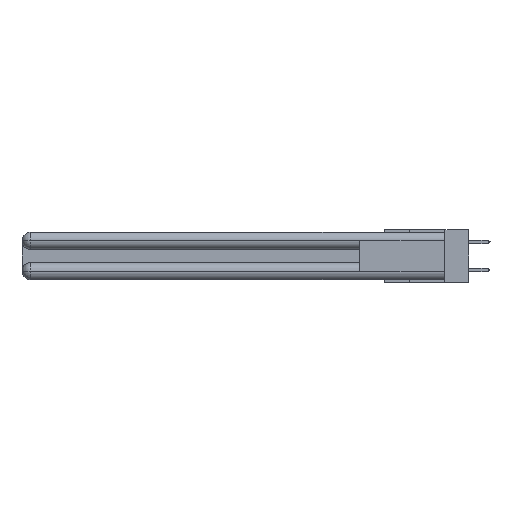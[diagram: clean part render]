
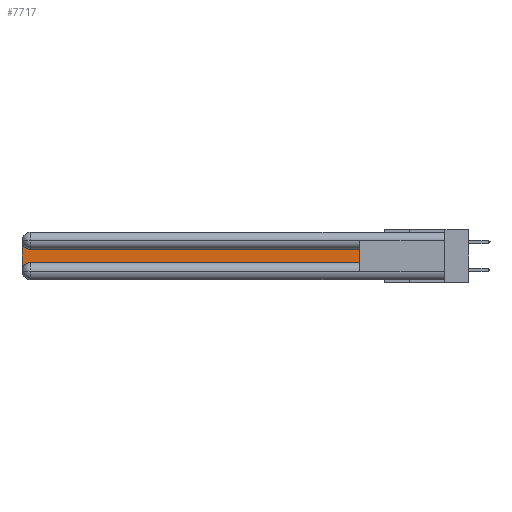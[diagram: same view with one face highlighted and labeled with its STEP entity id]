
A CAD part, left-side view. The second image highlights one B-rep face of the part: STEP entity #7717.
In plain terms, the highlighted planar face has unit normal (-1, 0, 0).
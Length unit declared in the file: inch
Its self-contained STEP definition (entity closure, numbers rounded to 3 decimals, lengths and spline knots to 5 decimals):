
#254 = DIRECTION ( 'NONE',  ( 0., 0., -1. ) ) ;
#842 = VECTOR ( 'NONE', #1793, 39.37008 ) ;
#943 = VERTEX_POINT ( 'NONE', #5503 ) ;
#1793 = DIRECTION ( 'NONE',  ( 0., 0., 1. ) ) ;
#3448 = CARTESIAN_POINT ( 'NONE',  ( 0.075, 0.6, -0.2175 ) ) ;
#3999 = DIRECTION ( 'NONE',  ( 0., 1., 0. ) ) ;
#5503 = CARTESIAN_POINT ( 'NONE',  ( 0.075, 0.6, -0.1225 ) ) ;
#5796 = DIRECTION ( 'NONE',  ( 0., 0., -1. ) ) ;
#7717 = ADVANCED_FACE ( 'NONE', ( #32579 ), #22457, .F. ) ;
#8227 = ORIENTED_EDGE ( 'NONE', *, *, #26157, .T. ) ;
#8641 = VECTOR ( 'NONE', #36005, 39.37008 ) ;
#8813 = AXIS2_PLACEMENT_3D ( 'NONE', #33532, #16880, #254 ) ;
#9236 = VERTEX_POINT ( 'NONE', #13924 ) ;
#10977 = VERTEX_POINT ( 'NONE', #3448 ) ;
#12655 = ORIENTED_EDGE ( 'NONE', *, *, #34220, .T. ) ;
#13216 = AXIS2_PLACEMENT_3D ( 'NONE', #22332, #30378, #13701 ) ;
#13701 = DIRECTION ( 'NONE',  ( 0., 0., -1. ) ) ;
#13829 = CARTESIAN_POINT ( 'NONE',  ( 0.075, 3., -0.1225 ) ) ;
#13924 = CARTESIAN_POINT ( 'NONE',  ( 0.075, 2.94, -0.1225 ) ) ;
#15434 = LINE ( 'NONE', #25744, #21072 ) ;
#16880 = DIRECTION ( 'NONE',  ( 1., 0., 0. ) ) ;
#17345 = CIRCLE ( 'NONE', #13216, 0.06 ) ;
#17694 = ORIENTED_EDGE ( 'NONE', *, *, #28349, .T. ) ;
#17769 = CARTESIAN_POINT ( 'NONE',  ( 0.075, 0.6, -0.1225 ) ) ;
#18044 = ORIENTED_EDGE ( 'NONE', *, *, #28180, .T. ) ;
#21072 = VECTOR ( 'NONE', #29280, 39.37008 ) ;
#21282 = EDGE_CURVE ( 'NONE', #943, #9236, #22815, .T. ) ;
#22332 = CARTESIAN_POINT ( 'NONE',  ( 0.075, 2.94, -0.0625 ) ) ;
#22457 = PLANE ( 'NONE',  #26092 ) ;
#22496 = EDGE_LOOP ( 'NONE', ( #29863, #31374, #17694, #18044, #12655, #8227 ) ) ;
#22815 = LINE ( 'NONE', #17769, #26358 ) ;
#24293 = CARTESIAN_POINT ( 'NONE',  ( 0.075, 3., -0.2775 ) ) ;
#24363 = EDGE_CURVE ( 'NONE', #9236, #33035, #17345, .T. ) ;
#24895 = CARTESIAN_POINT ( 'NONE',  ( 0.075, 0.6, -0.2175 ) ) ;
#25744 = CARTESIAN_POINT ( 'NONE',  ( 0.075, 3., -0.2175 ) ) ;
#26092 = AXIS2_PLACEMENT_3D ( 'NONE', #13829, #27825, #5796 ) ;
#26157 = EDGE_CURVE ( 'NONE', #10977, #943, #28646, .T. ) ;
#26358 = VECTOR ( 'NONE', #3999, 39.37008 ) ;
#26437 = CARTESIAN_POINT ( 'NONE',  ( 0.075, 0.6, -0.2175 ) ) ;
#27204 = CARTESIAN_POINT ( 'NONE',  ( 0.075, 3., -0.0625 ) ) ;
#27825 = DIRECTION ( 'NONE',  ( 1., 0., 0. ) ) ;
#28180 = EDGE_CURVE ( 'NONE', #31485, #33510, #35901, .T. ) ;
#28349 = EDGE_CURVE ( 'NONE', #33035, #31485, #15434, .T. ) ;
#28646 = LINE ( 'NONE', #26437, #842 ) ;
#29280 = DIRECTION ( 'NONE',  ( 0., 0., -1. ) ) ;
#29863 = ORIENTED_EDGE ( 'NONE', *, *, #21282, .T. ) ;
#30378 = DIRECTION ( 'NONE',  ( 1., 0., 0. ) ) ;
#31339 = CARTESIAN_POINT ( 'NONE',  ( 0.075, 2.94, -0.2175 ) ) ;
#31374 = ORIENTED_EDGE ( 'NONE', *, *, #24363, .T. ) ;
#31485 = VERTEX_POINT ( 'NONE', #24293 ) ;
#32579 = FACE_OUTER_BOUND ( 'NONE', #22496, .T. ) ;
#33035 = VERTEX_POINT ( 'NONE', #27204 ) ;
#33510 = VERTEX_POINT ( 'NONE', #31339 ) ;
#33532 = CARTESIAN_POINT ( 'NONE',  ( 0.075, 2.94, -0.2775 ) ) ;
#34220 = EDGE_CURVE ( 'NONE', #33510, #10977, #35651, .T. ) ;
#35651 = LINE ( 'NONE', #24895, #8641 ) ;
#35901 = CIRCLE ( 'NONE', #8813, 0.06 ) ;
#36005 = DIRECTION ( 'NONE',  ( 0., -1., 0. ) ) ;
